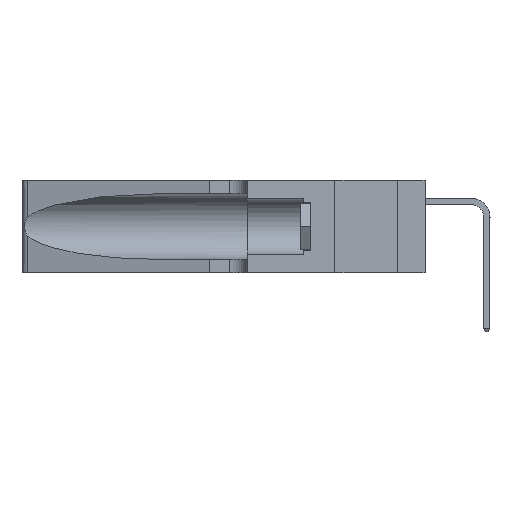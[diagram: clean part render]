
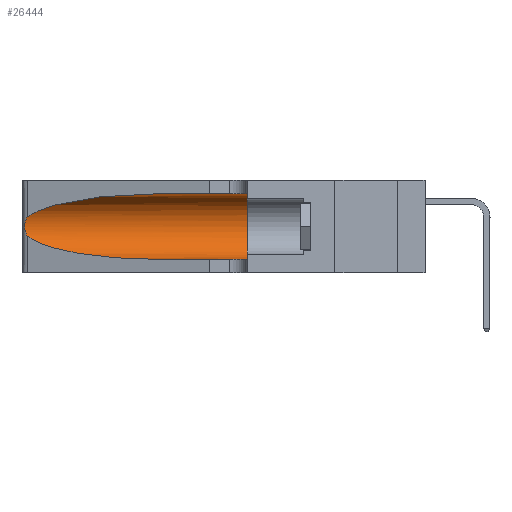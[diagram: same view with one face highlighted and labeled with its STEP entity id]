
A CAD part, left-side view. The second image highlights one B-rep face of the part: STEP entity #26444.
In plain terms, the highlighted cylindrical face has radius 3.308 mm (diameter 6.617 mm), a partial arc.
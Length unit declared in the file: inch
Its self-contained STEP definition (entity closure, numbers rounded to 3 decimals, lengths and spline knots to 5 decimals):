
#2509 =( BOUNDED_CURVE ( )  B_SPLINE_CURVE ( 3, ( #49151, #18245, #29893, #6752 ),
 .UNSPECIFIED., .F., .T. ) 
 B_SPLINE_CURVE_WITH_KNOTS ( ( 4, 4 ),
 ( 3.44316, 4.71239 ),
 .UNSPECIFIED. ) 
 CURVE ( )  GEOMETRIC_REPRESENTATION_ITEM ( )  RATIONAL_B_SPLINE_CURVE ( ( 1., 0.87, 0.87, 1. ) ) 
 REPRESENTATION_ITEM ( '' )  );
#2586 = CYLINDRICAL_SURFACE ( 'NONE', #20440, 0.13025 ) ;
#2627 = CARTESIAN_POINT ( 'NONE',  ( 0.1305, 0.72297, 0.31525 ) ) ;
#2728 = CARTESIAN_POINT ( 'NONE',  ( 0.25639, 1.23186, 0.15144 ) ) ;
#3557 = DIRECTION ( 'NONE',  ( 0., 0., -1. ) ) ;
#5259 =( BOUNDED_CURVE ( )  B_SPLINE_CURVE ( 3, ( #2627, #41376, #22031, #49096 ),
 .UNSPECIFIED., .F., .F. ) 
 B_SPLINE_CURVE_WITH_KNOTS ( ( 4, 4 ),
 ( 1.5708, 2.84003 ),
 .UNSPECIFIED. ) 
 CURVE ( )  GEOMETRIC_REPRESENTATION_ITEM ( )  RATIONAL_B_SPLINE_CURVE ( ( 1., 0.87, 0.87, 1. ) ) 
 REPRESENTATION_ITEM ( '' )  );
#6457 = CARTESIAN_POINT ( 'NONE',  ( 0.25487, 1.22718, 0.22369 ) ) ;
#6629 = CARTESIAN_POINT ( 'NONE',  ( 0.25487, 1.22718, 0.14631 ) ) ;
#6752 = CARTESIAN_POINT ( 'NONE',  ( 0.1305, 0.72297, 0.05475 ) ) ;
#7298 = VERTEX_POINT ( 'NONE', #11890 ) ;
#7810 = CARTESIAN_POINT ( 'NONE',  ( 0.1305, 0.35, 0.31525 ) ) ;
#8579 = CARTESIAN_POINT ( 'NONE',  ( 0.1305, 0.35, 0.185 ) ) ;
#10347 = CARTESIAN_POINT ( 'NONE',  ( 0.25639, 1.23184, 0.21858 ) ) ;
#10572 = DIRECTION ( 'NONE',  ( 0., -1., 0. ) ) ;
#11841 = VERTEX_POINT ( 'NONE', #22992 ) ;
#11890 = CARTESIAN_POINT ( 'NONE',  ( 0.25487, 1.22718, 0.22369 ) ) ;
#12062 = ORIENTED_EDGE ( 'NONE', *, *, #38891, .T. ) ;
#12464 = DIRECTION ( 'NONE',  ( 0., 0., 1. ) ) ;
#14226 = CARTESIAN_POINT ( 'NONE',  ( 0.25854, 1.2359, 0.20912 ) ) ;
#14392 = AXIS2_PLACEMENT_3D ( 'NONE', #8579, #35623, #12464 ) ;
#16186 = ORIENTED_EDGE ( 'NONE', *, *, #37191, .T. ) ;
#17167 = LINE ( 'NONE', #37648, #36514 ) ;
#18126 = CARTESIAN_POINT ( 'NONE',  ( 0.26075, 1.23896, 0.19203 ) ) ;
#18245 = CARTESIAN_POINT ( 'NONE',  ( 0.2373, 1.15595, 0.08982 ) ) ;
#20440 = AXIS2_PLACEMENT_3D ( 'NONE', #42275, #38383, #3557 ) ;
#20680 = B_SPLINE_CURVE_WITH_KNOTS ( 'NONE', 3,
 ( #6457, #25689, #10347, #37407, #14226, #41312, #18126, #45167, #21968, #49029, #25865, #2728, #29780, #6629 ),
 .UNSPECIFIED., .F., .F.,
 ( 4, 2, 2, 2, 2, 2, 4 ),
 ( 0., 0.00027, 0.00053, 0.00107, 0.0016, 0.00187, 0.00214 ),
 .UNSPECIFIED. ) ;
#20848 = CIRCLE ( 'NONE', #14392, 0.13025 ) ;
#21968 = CARTESIAN_POINT ( 'NONE',  ( 0.26017, 1.23833, 0.17102 ) ) ;
#22031 = CARTESIAN_POINT ( 'NONE',  ( 0.2373, 1.15595, 0.28018 ) ) ;
#22992 = CARTESIAN_POINT ( 'NONE',  ( 0.25487, 1.22718, 0.14631 ) ) ;
#23335 = CARTESIAN_POINT ( 'NONE',  ( 0.1305, 0.72297, 0.05475 ) ) ;
#24050 = VERTEX_POINT ( 'NONE', #32877 ) ;
#25263 = ORIENTED_EDGE ( 'NONE', *, *, #37646, .F. ) ;
#25592 = CARTESIAN_POINT ( 'NONE',  ( 0.1305, 0.35, 0.05475 ) ) ;
#25689 = CARTESIAN_POINT ( 'NONE',  ( 0.25555, 1.22994, 0.2215 ) ) ;
#25865 = CARTESIAN_POINT ( 'NONE',  ( 0.25789, 1.23486, 0.15765 ) ) ;
#26237 = VECTOR ( 'NONE', #34712, 39.37008 ) ;
#26444 = ADVANCED_FACE ( 'NONE', ( #33435 ), #2586, .F. ) ;
#27476 = LINE ( 'NONE', #30854, #26237 ) ;
#28542 = ORIENTED_EDGE ( 'NONE', *, *, #46152, .T. ) ;
#29780 = CARTESIAN_POINT ( 'NONE',  ( 0.25555, 1.22993, 0.14849 ) ) ;
#29893 = CARTESIAN_POINT ( 'NONE',  ( 0.18966, 0.96281, 0.05475 ) ) ;
#30202 = ORIENTED_EDGE ( 'NONE', *, *, #36718, .F. ) ;
#30854 = CARTESIAN_POINT ( 'NONE',  ( 0.1305, 1.61858, 0.05475 ) ) ;
#32877 = CARTESIAN_POINT ( 'NONE',  ( 0.1305, 0.72297, 0.31525 ) ) ;
#33435 = FACE_OUTER_BOUND ( 'NONE', #46743, .T. ) ;
#34712 = DIRECTION ( 'NONE',  ( 0., -1., 0. ) ) ;
#35623 = DIRECTION ( 'NONE',  ( 0., 1., 0. ) ) ;
#35873 = VERTEX_POINT ( 'NONE', #7810 ) ;
#36514 = VECTOR ( 'NONE', #10572, 39.37008 ) ;
#36718 = EDGE_CURVE ( 'NONE', #35873, #48776, #20848, .T. ) ;
#37018 = EDGE_CURVE ( 'NONE', #24050, #7298, #5259, .T. ) ;
#37191 = EDGE_CURVE ( 'NONE', #40761, #48776, #27476, .T. ) ;
#37407 = CARTESIAN_POINT ( 'NONE',  ( 0.25787, 1.23484, 0.2124 ) ) ;
#37646 = EDGE_CURVE ( 'NONE', #24050, #35873, #17167, .T. ) ;
#37648 = CARTESIAN_POINT ( 'NONE',  ( 0.1305, 1.61858, 0.31525 ) ) ;
#38383 = DIRECTION ( 'NONE',  ( 0., -1., 0. ) ) ;
#38891 = EDGE_CURVE ( 'NONE', #11841, #40761, #2509, .T. ) ;
#40761 = VERTEX_POINT ( 'NONE', #23335 ) ;
#41312 = CARTESIAN_POINT ( 'NONE',  ( 0.26018, 1.23835, 0.19895 ) ) ;
#41376 = CARTESIAN_POINT ( 'NONE',  ( 0.18966, 0.96281, 0.31525 ) ) ;
#42275 = CARTESIAN_POINT ( 'NONE',  ( 0.1305, 1.61858, 0.185 ) ) ;
#44540 = ORIENTED_EDGE ( 'NONE', *, *, #37018, .T. ) ;
#45167 = CARTESIAN_POINT ( 'NONE',  ( 0.26075, 1.23896, 0.178 ) ) ;
#46152 = EDGE_CURVE ( 'NONE', #7298, #11841, #20680, .T. ) ;
#46743 = EDGE_LOOP ( 'NONE', ( #44540, #28542, #12062, #16186, #30202, #25263 ) ) ;
#48776 = VERTEX_POINT ( 'NONE', #25592 ) ;
#49029 = CARTESIAN_POINT ( 'NONE',  ( 0.25856, 1.23593, 0.16098 ) ) ;
#49096 = CARTESIAN_POINT ( 'NONE',  ( 0.25487, 1.22718, 0.22369 ) ) ;
#49151 = CARTESIAN_POINT ( 'NONE',  ( 0.25487, 1.22718, 0.14631 ) ) ;
